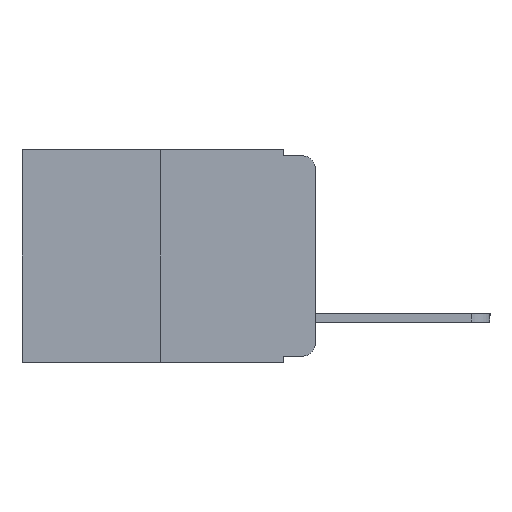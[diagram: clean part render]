
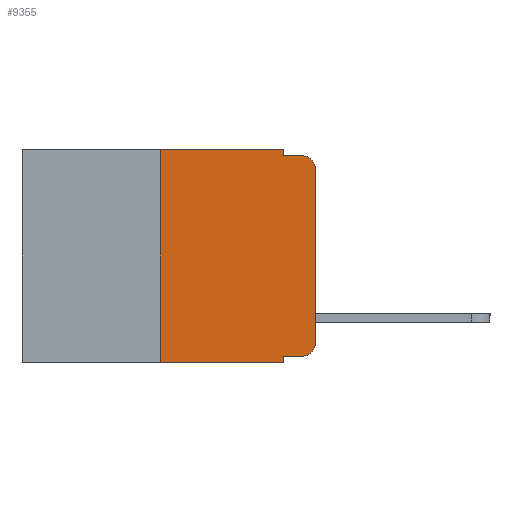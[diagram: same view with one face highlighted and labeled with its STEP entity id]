
A CAD part, left-side view. The second image highlights one B-rep face of the part: STEP entity #9355.
In plain terms, the highlighted planar face has unit normal (-1, 0, 0).
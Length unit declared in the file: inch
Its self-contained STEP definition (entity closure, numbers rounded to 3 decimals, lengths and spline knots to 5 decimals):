
#136 = VECTOR ( 'NONE', #7534, 39.37008 ) ;
#208 = EDGE_CURVE ( 'NONE', #5412, #12739, #8009, .T. ) ;
#317 = VERTEX_POINT ( 'NONE', #11538 ) ;
#341 = VECTOR ( 'NONE', #16781, 39.37008 ) ;
#572 = CARTESIAN_POINT ( 'NONE',  ( 0., 0.02, -0.313 ) ) ;
#830 = EDGE_CURVE ( 'NONE', #19893, #3088, #15838, .T. ) ;
#961 = CARTESIAN_POINT ( 'NONE',  ( 0., 0.473, 0. ) ) ;
#2170 = DIRECTION ( 'NONE',  ( 0., 0., -1. ) ) ;
#2560 = EDGE_CURVE ( 'NONE', #19893, #14485, #3805, .T. ) ;
#2888 = VECTOR ( 'NONE', #11270, 39.37008 ) ;
#3088 = VERTEX_POINT ( 'NONE', #17981 ) ;
#3303 = VECTOR ( 'NONE', #8511, 39.37008 ) ;
#3573 = AXIS2_PLACEMENT_3D ( 'NONE', #961, #16555, #7239 ) ;
#3805 = LINE ( 'NONE', #16835, #136 ) ;
#4321 = CARTESIAN_POINT ( 'NONE',  ( 0., 0.051, -0.01 ) ) ;
#4592 = CARTESIAN_POINT ( 'NONE',  ( 0., 0.051, -0.333 ) ) ;
#4889 = EDGE_CURVE ( 'NONE', #6938, #3088, #15748, .T. ) ;
#5412 = VERTEX_POINT ( 'NONE', #8132 ) ;
#5670 = PLANE ( 'NONE',  #3573 ) ;
#5773 = ORIENTED_EDGE ( 'NONE', *, *, #10038, .T. ) ;
#5799 = CARTESIAN_POINT ( 'NONE',  ( 0., 0.25, 0. ) ) ;
#5909 = CARTESIAN_POINT ( 'NONE',  ( 0., 0.473, 0. ) ) ;
#6061 = ORIENTED_EDGE ( 'NONE', *, *, #13188, .T. ) ;
#6084 = ORIENTED_EDGE ( 'NONE', *, *, #11080, .F. ) ;
#6237 = ORIENTED_EDGE ( 'NONE', *, *, #208, .F. ) ;
#6452 = EDGE_CURVE ( 'NONE', #14485, #15536, #16208, .T. ) ;
#6464 = EDGE_LOOP ( 'NONE', ( #5773, #6061, #6084, #6237, #7000, #7058, #7729, #7680, #10342, #8844 ) ) ;
#6696 = EDGE_CURVE ( 'NONE', #7876, #5412, #7173, .T. ) ;
#6757 = CIRCLE ( 'NONE', #8996, 0.02 ) ;
#6937 = CARTESIAN_POINT ( 'NONE',  ( 0., 0.473, -0.343 ) ) ;
#6938 = VERTEX_POINT ( 'NONE', #14255 ) ;
#7000 = ORIENTED_EDGE ( 'NONE', *, *, #6696, .F. ) ;
#7058 = ORIENTED_EDGE ( 'NONE', *, *, #14283, .F. ) ;
#7173 = LINE ( 'NONE', #5909, #341 ) ;
#7239 = DIRECTION ( 'NONE',  ( 0., 0., -1. ) ) ;
#7534 = DIRECTION ( 'NONE',  ( 0., -1., 0. ) ) ;
#7680 = ORIENTED_EDGE ( 'NONE', *, *, #830, .F. ) ;
#7729 = ORIENTED_EDGE ( 'NONE', *, *, #4889, .T. ) ;
#7876 = VERTEX_POINT ( 'NONE', #5799 ) ;
#8009 = LINE ( 'NONE', #18881, #2888 ) ;
#8132 = CARTESIAN_POINT ( 'NONE',  ( 0., 0.051, 0. ) ) ;
#8511 = DIRECTION ( 'NONE',  ( 0., -1., 0. ) ) ;
#8546 = DIRECTION ( 'NONE',  ( -1., 0., 0. ) ) ;
#8844 = ORIENTED_EDGE ( 'NONE', *, *, #6452, .T. ) ;
#8996 = AXIS2_PLACEMENT_3D ( 'NONE', #17805, #8546, #19315 ) ;
#9128 = DIRECTION ( 'NONE',  ( 0., 0., 1. ) ) ;
#9355 = ADVANCED_FACE ( 'NONE', ( #15940 ), #5670, .F. ) ;
#9587 = DIRECTION ( 'NONE',  ( 0., 0., -1. ) ) ;
#10038 = EDGE_CURVE ( 'NONE', #15536, #16618, #17081, .T. ) ;
#10290 = DIRECTION ( 'NONE',  ( 0., 0., 1. ) ) ;
#10342 = ORIENTED_EDGE ( 'NONE', *, *, #2560, .T. ) ;
#10425 = VECTOR ( 'NONE', #10290, 39.37008 ) ;
#11080 = EDGE_CURVE ( 'NONE', #12739, #317, #14212, .T. ) ;
#11099 = CARTESIAN_POINT ( 'NONE',  ( 0., 0.051, 0. ) ) ;
#11270 = DIRECTION ( 'NONE',  ( 0., 0., -1. ) ) ;
#11538 = CARTESIAN_POINT ( 'NONE',  ( 0., 0.02, -0.01 ) ) ;
#11544 = DIRECTION ( 'NONE',  ( -1., 0., 0. ) ) ;
#11703 = DIRECTION ( 'NONE',  ( 0., -1., 0. ) ) ;
#12524 = VECTOR ( 'NONE', #9128, 39.37008 ) ;
#12739 = VERTEX_POINT ( 'NONE', #4321 ) ;
#13188 = EDGE_CURVE ( 'NONE', #16618, #317, #6757, .T. ) ;
#13232 = VECTOR ( 'NONE', #11703, 39.37008 ) ;
#13295 = CARTESIAN_POINT ( 'NONE',  ( 0., 0.051, -0.01 ) ) ;
#13907 = CARTESIAN_POINT ( 'NONE',  ( 0., 0.02, -0.333 ) ) ;
#14169 = AXIS2_PLACEMENT_3D ( 'NONE', #572, #11544, #2170 ) ;
#14212 = LINE ( 'NONE', #13295, #13232 ) ;
#14255 = CARTESIAN_POINT ( 'NONE',  ( 0., 0.25, -0.343 ) ) ;
#14283 = EDGE_CURVE ( 'NONE', #6938, #7876, #18564, .T. ) ;
#14485 = VERTEX_POINT ( 'NONE', #13907 ) ;
#15218 = CARTESIAN_POINT ( 'NONE',  ( 0., 0., -0.313 ) ) ;
#15363 = VECTOR ( 'NONE', #9587, 39.37008 ) ;
#15536 = VERTEX_POINT ( 'NONE', #15218 ) ;
#15748 = LINE ( 'NONE', #6937, #3303 ) ;
#15838 = LINE ( 'NONE', #11099, #15363 ) ;
#15940 = FACE_OUTER_BOUND ( 'NONE', #6464, .T. ) ;
#16208 = CIRCLE ( 'NONE', #14169, 0.02 ) ;
#16555 = DIRECTION ( 'NONE',  ( 1., 0., 0. ) ) ;
#16618 = VERTEX_POINT ( 'NONE', #17800 ) ;
#16781 = DIRECTION ( 'NONE',  ( 0., -1., 0. ) ) ;
#16835 = CARTESIAN_POINT ( 'NONE',  ( 0., 0.051, -0.333 ) ) ;
#17081 = LINE ( 'NONE', #18357, #12524 ) ;
#17800 = CARTESIAN_POINT ( 'NONE',  ( 0., 0., -0.03 ) ) ;
#17805 = CARTESIAN_POINT ( 'NONE',  ( 0., 0.02, -0.03 ) ) ;
#17981 = CARTESIAN_POINT ( 'NONE',  ( 0., 0.051, -0.343 ) ) ;
#18357 = CARTESIAN_POINT ( 'NONE',  ( 0., 0., 0. ) ) ;
#18564 = LINE ( 'NONE', #19468, #10425 ) ;
#18881 = CARTESIAN_POINT ( 'NONE',  ( 0., 0.051, 0. ) ) ;
#19315 = DIRECTION ( 'NONE',  ( 0., 0., -1. ) ) ;
#19468 = CARTESIAN_POINT ( 'NONE',  ( 0., 0.25, 0. ) ) ;
#19893 = VERTEX_POINT ( 'NONE', #4592 ) ;
